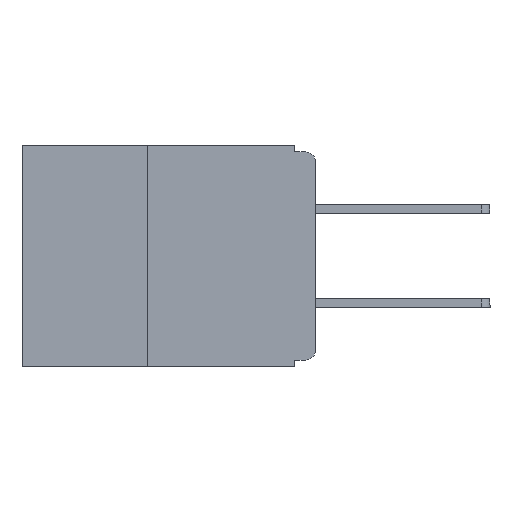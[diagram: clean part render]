
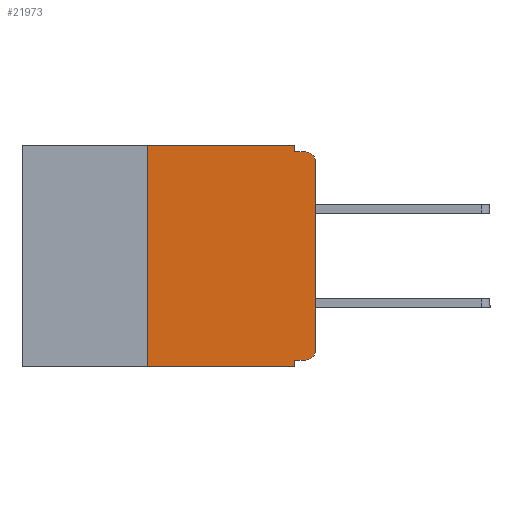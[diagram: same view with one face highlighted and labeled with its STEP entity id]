
A CAD part, left-side view. The second image highlights one B-rep face of the part: STEP entity #21973.
In plain terms, the highlighted planar face has unit normal (-1, 0, 0).
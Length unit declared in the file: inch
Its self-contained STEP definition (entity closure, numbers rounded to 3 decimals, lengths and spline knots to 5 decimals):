
#138 = VECTOR ( 'NONE', #23488, 39.37008 ) ;
#378 = CARTESIAN_POINT ( 'NONE',  ( 0., 0.437, -0.33 ) ) ;
#887 = CARTESIAN_POINT ( 'NONE',  ( 0., 0., -0.025 ) ) ;
#1519 = VERTEX_POINT ( 'NONE', #2689 ) ;
#1629 = FACE_OUTER_BOUND ( 'NONE', #21701, .T. ) ;
#1662 = VERTEX_POINT ( 'NONE', #17099 ) ;
#1854 = EDGE_CURVE ( 'NONE', #20796, #27883, #19620, .T. ) ;
#2079 = CIRCLE ( 'NONE', #6094, 0.015 ) ;
#2249 = ORIENTED_EDGE ( 'NONE', *, *, #13418, .T. ) ;
#2689 = CARTESIAN_POINT ( 'NONE',  ( 0., 0.031, -0.32 ) ) ;
#3581 = ORIENTED_EDGE ( 'NONE', *, *, #9325, .F. ) ;
#3682 = CARTESIAN_POINT ( 'NONE',  ( 0., 0.015, -0.305 ) ) ;
#3732 = EDGE_CURVE ( 'NONE', #20796, #1519, #9151, .T. ) ;
#3837 = DIRECTION ( 'NONE',  ( -1., 0., 0. ) ) ;
#3885 = LINE ( 'NONE', #19832, #9075 ) ;
#4270 = VECTOR ( 'NONE', #22255, 39.37008 ) ;
#5653 = VERTEX_POINT ( 'NONE', #19741 ) ;
#5690 = EDGE_CURVE ( 'NONE', #18000, #5653, #3885, .T. ) ;
#5917 = VERTEX_POINT ( 'NONE', #887 ) ;
#5993 = LINE ( 'NONE', #14774, #138 ) ;
#6094 = AXIS2_PLACEMENT_3D ( 'NONE', #24213, #11132, #26363 ) ;
#6672 = VERTEX_POINT ( 'NONE', #8373 ) ;
#6748 = ORIENTED_EDGE ( 'NONE', *, *, #1854, .T. ) ;
#6928 = CARTESIAN_POINT ( 'NONE',  ( 0., 0.031, -0.33 ) ) ;
#7236 = ORIENTED_EDGE ( 'NONE', *, *, #20085, .T. ) ;
#7694 = ORIENTED_EDGE ( 'NONE', *, *, #3732, .F. ) ;
#8076 = DIRECTION ( 'NONE',  ( 0., 0., -1. ) ) ;
#8373 = CARTESIAN_POINT ( 'NONE',  ( 0., 0.015, -0.01 ) ) ;
#8472 = VECTOR ( 'NONE', #21906, 39.37008 ) ;
#8496 = LINE ( 'NONE', #21950, #23863 ) ;
#8807 = CARTESIAN_POINT ( 'NONE',  ( 0., 0., -0.01 ) ) ;
#9075 = VECTOR ( 'NONE', #22004, 39.37008 ) ;
#9151 = LINE ( 'NONE', #16175, #24509 ) ;
#9162 = LINE ( 'NONE', #8807, #8472 ) ;
#9306 = ORIENTED_EDGE ( 'NONE', *, *, #24385, .T. ) ;
#9325 = EDGE_CURVE ( 'NONE', #1662, #6672, #9162, .T. ) ;
#9503 = CARTESIAN_POINT ( 'NONE',  ( 0., 0.015, -0.32 ) ) ;
#9634 = ORIENTED_EDGE ( 'NONE', *, *, #23304, .F. ) ;
#10204 = CARTESIAN_POINT ( 'NONE',  ( 0., 0.25, 0. ) ) ;
#11132 = DIRECTION ( 'NONE',  ( -1., 0., 0. ) ) ;
#11952 = VERTEX_POINT ( 'NONE', #12556 ) ;
#12070 = CARTESIAN_POINT ( 'NONE',  ( 0., 0.25, -0.33 ) ) ;
#12556 = CARTESIAN_POINT ( 'NONE',  ( 0., 0.031, -0.33 ) ) ;
#12649 = LINE ( 'NONE', #378, #17759 ) ;
#13418 = EDGE_CURVE ( 'NONE', #5917, #6672, #2079, .T. ) ;
#13553 = LINE ( 'NONE', #18887, #18651 ) ;
#14774 = CARTESIAN_POINT ( 'NONE',  ( 0., 0.25, -0.33 ) ) ;
#16087 = DIRECTION ( 'NONE',  ( 0., 1., 0. ) ) ;
#16175 = CARTESIAN_POINT ( 'NONE',  ( 0., 0., -0.32 ) ) ;
#17099 = CARTESIAN_POINT ( 'NONE',  ( 0., 0.031, -0.01 ) ) ;
#17759 = VECTOR ( 'NONE', #17980, 39.37008 ) ;
#17980 = DIRECTION ( 'NONE',  ( 0., -1., 0. ) ) ;
#18000 = VERTEX_POINT ( 'NONE', #10204 ) ;
#18651 = VECTOR ( 'NONE', #18791, 39.37008 ) ;
#18791 = DIRECTION ( 'NONE',  ( 0., 0., 1. ) ) ;
#18887 = CARTESIAN_POINT ( 'NONE',  ( 0., 0., 0. ) ) ;
#19022 = PLANE ( 'NONE',  #21119 ) ;
#19620 = CIRCLE ( 'NONE', #27414, 0.015 ) ;
#19741 = CARTESIAN_POINT ( 'NONE',  ( 0., 0.031, 0. ) ) ;
#19777 = DIRECTION ( 'NONE',  ( 0., 0., -1. ) ) ;
#19832 = CARTESIAN_POINT ( 'NONE',  ( 0., 0.437, 0. ) ) ;
#20085 = EDGE_CURVE ( 'NONE', #23164, #11952, #12649, .T. ) ;
#20796 = VERTEX_POINT ( 'NONE', #9503 ) ;
#20832 = DIRECTION ( 'NONE',  ( 0., 0., -1. ) ) ;
#21119 = AXIS2_PLACEMENT_3D ( 'NONE', #23276, #21198, #8076 ) ;
#21198 = DIRECTION ( 'NONE',  ( 1., 0., 0. ) ) ;
#21701 = EDGE_LOOP ( 'NONE', ( #9306, #2249, #3581, #25442, #24660, #9634, #7236, #24919, #7694, #6748 ) ) ;
#21759 = LINE ( 'NONE', #6928, #4270 ) ;
#21906 = DIRECTION ( 'NONE',  ( 0., -1., 0. ) ) ;
#21950 = CARTESIAN_POINT ( 'NONE',  ( 0., 0.031, 0. ) ) ;
#21973 = ADVANCED_FACE ( 'NONE', ( #1629 ), #19022, .F. ) ;
#22004 = DIRECTION ( 'NONE',  ( 0., -1., 0. ) ) ;
#22198 = EDGE_CURVE ( 'NONE', #5653, #1662, #8496, .T. ) ;
#22255 = DIRECTION ( 'NONE',  ( 0., 0., -1. ) ) ;
#23164 = VERTEX_POINT ( 'NONE', #12070 ) ;
#23276 = CARTESIAN_POINT ( 'NONE',  ( 0., 0.437, 0. ) ) ;
#23304 = EDGE_CURVE ( 'NONE', #23164, #18000, #5993, .T. ) ;
#23488 = DIRECTION ( 'NONE',  ( 0., 0., 1. ) ) ;
#23557 = EDGE_CURVE ( 'NONE', #1519, #11952, #21759, .T. ) ;
#23863 = VECTOR ( 'NONE', #19777, 39.37008 ) ;
#24213 = CARTESIAN_POINT ( 'NONE',  ( 0., 0.015, -0.025 ) ) ;
#24385 = EDGE_CURVE ( 'NONE', #27883, #5917, #13553, .T. ) ;
#24509 = VECTOR ( 'NONE', #16087, 39.37008 ) ;
#24660 = ORIENTED_EDGE ( 'NONE', *, *, #5690, .F. ) ;
#24919 = ORIENTED_EDGE ( 'NONE', *, *, #23557, .F. ) ;
#25442 = ORIENTED_EDGE ( 'NONE', *, *, #22198, .F. ) ;
#26363 = DIRECTION ( 'NONE',  ( 0., 0., -1. ) ) ;
#26474 = CARTESIAN_POINT ( 'NONE',  ( 0., 0., -0.305 ) ) ;
#27414 = AXIS2_PLACEMENT_3D ( 'NONE', #3682, #3837, #20832 ) ;
#27883 = VERTEX_POINT ( 'NONE', #26474 ) ;
